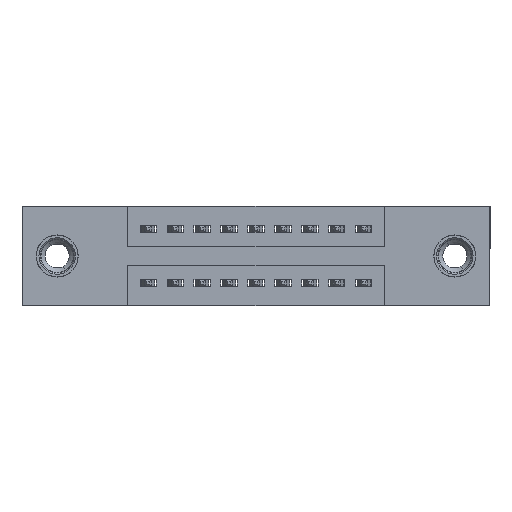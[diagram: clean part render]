
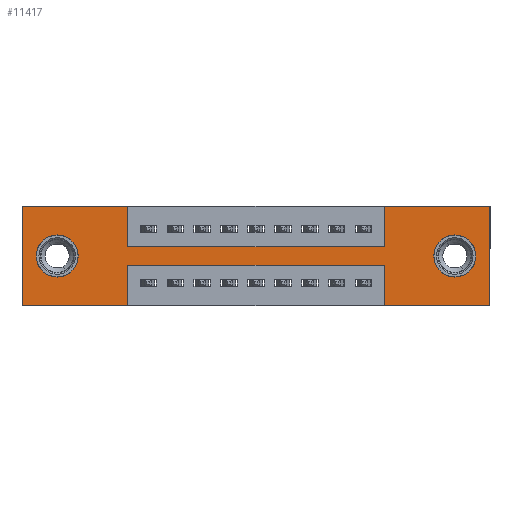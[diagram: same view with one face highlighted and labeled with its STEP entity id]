
A CAD part, front view. The second image highlights one B-rep face of the part: STEP entity #11417.
In plain terms, the highlighted planar face has unit normal (0, -1, 0).
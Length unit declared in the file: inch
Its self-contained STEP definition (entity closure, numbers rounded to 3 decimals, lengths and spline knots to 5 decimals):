
#374 = CARTESIAN_POINT ( 'NONE',  ( 0.13, 0., -0.263 ) ) ;
#575 = VERTEX_POINT ( 'NONE', #3489 ) ;
#651 = VERTEX_POINT ( 'NONE', #3044 ) ;
#823 = VERTEX_POINT ( 'NONE', #2618 ) ;
#985 = CARTESIAN_POINT ( 'NONE',  ( 1.3425, 0., 0. ) ) ;
#1018 = EDGE_CURVE ( 'NONE', #11412, #2988, #15150, .T. ) ;
#1039 = VERTEX_POINT ( 'NONE', #2217 ) ;
#1085 = EDGE_LOOP ( 'NONE', ( #7221, #8420 ) ) ;
#1152 = LINE ( 'NONE', #8568, #4815 ) ;
#1258 = CARTESIAN_POINT ( 'NONE',  ( 0., 0., -0.37 ) ) ;
#1342 = DIRECTION ( 'NONE',  ( 0., 0., 1. ) ) ;
#1344 = VERTEX_POINT ( 'NONE', #10447 ) ;
#1392 = DIRECTION ( 'NONE',  ( 0., 0., 1. ) ) ;
#1955 = VECTOR ( 'NONE', #10590, 39.37008 ) ;
#1995 = DIRECTION ( 'NONE',  ( 0., 1., 0. ) ) ;
#2217 = CARTESIAN_POINT ( 'NONE',  ( 0.3925, 0., -0.22 ) ) ;
#2341 = VERTEX_POINT ( 'NONE', #6808 ) ;
#2471 = FACE_BOUND ( 'NONE', #9876, .T. ) ;
#2543 = VERTEX_POINT ( 'NONE', #8246 ) ;
#2618 = CARTESIAN_POINT ( 'NONE',  ( 0., 0., 0. ) ) ;
#2703 = ORIENTED_EDGE ( 'NONE', *, *, #6531, .F. ) ;
#2709 = VERTEX_POINT ( 'NONE', #1258 ) ;
#2840 = LINE ( 'NONE', #4169, #12489 ) ;
#2851 = LINE ( 'NONE', #6890, #1955 ) ;
#2918 = VERTEX_POINT ( 'NONE', #7575 ) ;
#2976 = CARTESIAN_POINT ( 'NONE',  ( 0., 0., -0.37 ) ) ;
#2988 = VERTEX_POINT ( 'NONE', #10136 ) ;
#3044 = CARTESIAN_POINT ( 'NONE',  ( 1.735, 0., -0.37 ) ) ;
#3046 = VECTOR ( 'NONE', #15604, 39.37008 ) ;
#3374 = ORIENTED_EDGE ( 'NONE', *, *, #14021, .F. ) ;
#3489 = CARTESIAN_POINT ( 'NONE',  ( 1.605, 0., -0.107 ) ) ;
#3557 = ORIENTED_EDGE ( 'NONE', *, *, #7075, .T. ) ;
#3801 = CARTESIAN_POINT ( 'NONE',  ( 0.13, 0., -0.107 ) ) ;
#4063 = DIRECTION ( 'NONE',  ( 0., 0., -1. ) ) ;
#4169 = CARTESIAN_POINT ( 'NONE',  ( 0.3925, 0., -0.15 ) ) ;
#4176 = ORIENTED_EDGE ( 'NONE', *, *, #16287, .F. ) ;
#4330 = DIRECTION ( 'NONE',  ( 0., -1., 0. ) ) ;
#4395 = EDGE_CURVE ( 'NONE', #823, #2918, #2851, .T. ) ;
#4518 = VERTEX_POINT ( 'NONE', #374 ) ;
#4541 = VECTOR ( 'NONE', #7752, 39.37008 ) ;
#4552 = VECTOR ( 'NONE', #16025, 39.37008 ) ;
#4579 = EDGE_CURVE ( 'NONE', #2988, #1344, #10290, .T. ) ;
#4738 = EDGE_CURVE ( 'NONE', #2709, #823, #8368, .T. ) ;
#4815 = VECTOR ( 'NONE', #11016, 39.37008 ) ;
#4863 = EDGE_CURVE ( 'NONE', #2543, #11412, #2840, .T. ) ;
#5030 = CARTESIAN_POINT ( 'NONE',  ( 1.605, 0., -0.185 ) ) ;
#5120 = EDGE_CURVE ( 'NONE', #9756, #575, #8960, .T. ) ;
#5175 = DIRECTION ( 'NONE',  ( 0., 1., 0. ) ) ;
#5252 = CARTESIAN_POINT ( 'NONE',  ( 0., 0., -0.37 ) ) ;
#5296 = VERTEX_POINT ( 'NONE', #3801 ) ;
#5560 = VERTEX_POINT ( 'NONE', #9362 ) ;
#6025 = FACE_OUTER_BOUND ( 'NONE', #12438, .T. ) ;
#6253 = DIRECTION ( 'NONE',  ( 0., 0., -1. ) ) ;
#6317 = DIRECTION ( 'NONE',  ( 0., 0., -1. ) ) ;
#6364 = CARTESIAN_POINT ( 'NONE',  ( 1.3425, 0., -0.22 ) ) ;
#6531 = EDGE_CURVE ( 'NONE', #1344, #651, #11244, .T. ) ;
#6646 = ORIENTED_EDGE ( 'NONE', *, *, #1018, .F. ) ;
#6764 = CIRCLE ( 'NONE', #14622, 0.078 ) ;
#6808 = CARTESIAN_POINT ( 'NONE',  ( 1.3425, 0., -0.37 ) ) ;
#6890 = CARTESIAN_POINT ( 'NONE',  ( 0., 0., 0. ) ) ;
#7075 = EDGE_CURVE ( 'NONE', #4518, #5296, #6764, .T. ) ;
#7105 = CARTESIAN_POINT ( 'NONE',  ( 0.3925, 0., -0.37 ) ) ;
#7206 = DIRECTION ( 'NONE',  ( 1., 0., 0. ) ) ;
#7221 = ORIENTED_EDGE ( 'NONE', *, *, #12921, .T. ) ;
#7358 = EDGE_CURVE ( 'NONE', #10042, #1039, #15397, .T. ) ;
#7440 = ORIENTED_EDGE ( 'NONE', *, *, #4863, .F. ) ;
#7575 = CARTESIAN_POINT ( 'NONE',  ( 0.3925, 0., 0. ) ) ;
#7644 = ORIENTED_EDGE ( 'NONE', *, *, #4395, .F. ) ;
#7707 = LINE ( 'NONE', #9992, #15546 ) ;
#7752 = DIRECTION ( 'NONE',  ( 0., 0., 1. ) ) ;
#7918 = VECTOR ( 'NONE', #4063, 39.37008 ) ;
#7976 = LINE ( 'NONE', #13678, #10875 ) ;
#8048 = VECTOR ( 'NONE', #13817, 39.37008 ) ;
#8246 = CARTESIAN_POINT ( 'NONE',  ( 0.3925, 0., -0.15 ) ) ;
#8368 = LINE ( 'NONE', #13741, #4541 ) ;
#8420 = ORIENTED_EDGE ( 'NONE', *, *, #5120, .T. ) ;
#8480 = CARTESIAN_POINT ( 'NONE',  ( 0., 0., 0. ) ) ;
#8520 = EDGE_CURVE ( 'NONE', #1039, #5560, #11551, .T. ) ;
#8568 = CARTESIAN_POINT ( 'NONE',  ( 1.3425, 0., -0.37 ) ) ;
#8854 = AXIS2_PLACEMENT_3D ( 'NONE', #2976, #4330, #12988 ) ;
#8889 = ORIENTED_EDGE ( 'NONE', *, *, #12377, .F. ) ;
#8955 = CARTESIAN_POINT ( 'NONE',  ( 1.735, 0., 0. ) ) ;
#8960 = CIRCLE ( 'NONE', #15353, 0.078 ) ;
#9217 = DIRECTION ( 'NONE',  ( 0., 1., 0. ) ) ;
#9362 = CARTESIAN_POINT ( 'NONE',  ( 0.3925, 0., -0.37 ) ) ;
#9600 = ORIENTED_EDGE ( 'NONE', *, *, #4579, .F. ) ;
#9633 = CARTESIAN_POINT ( 'NONE',  ( 1.605, 0., -0.263 ) ) ;
#9756 = VERTEX_POINT ( 'NONE', #9633 ) ;
#9800 = CARTESIAN_POINT ( 'NONE',  ( 1.605, 0., -0.185 ) ) ;
#9876 = EDGE_LOOP ( 'NONE', ( #15468, #3557 ) ) ;
#9992 = CARTESIAN_POINT ( 'NONE',  ( 0.3925, 0., 0. ) ) ;
#10042 = VERTEX_POINT ( 'NONE', #6364 ) ;
#10136 = CARTESIAN_POINT ( 'NONE',  ( 1.3425, 0., 0. ) ) ;
#10290 = LINE ( 'NONE', #8480, #13044 ) ;
#10393 = EDGE_CURVE ( 'NONE', #2341, #10042, #1152, .T. ) ;
#10447 = CARTESIAN_POINT ( 'NONE',  ( 1.735, 0., 0. ) ) ;
#10590 = DIRECTION ( 'NONE',  ( 1., 0., 0. ) ) ;
#10650 = PLANE ( 'NONE',  #8854 ) ;
#10735 = ORIENTED_EDGE ( 'NONE', *, *, #8520, .F. ) ;
#10875 = VECTOR ( 'NONE', #12507, 39.37008 ) ;
#11016 = DIRECTION ( 'NONE',  ( 0., 0., 1. ) ) ;
#11050 = DIRECTION ( 'NONE',  ( 0., 0., -1. ) ) ;
#11117 = ORIENTED_EDGE ( 'NONE', *, *, #7358, .F. ) ;
#11244 = LINE ( 'NONE', #8955, #4552 ) ;
#11412 = VERTEX_POINT ( 'NONE', #14148 ) ;
#11417 = ADVANCED_FACE ( 'NONE', ( #15648, #2471, #6025 ), #10650, .T. ) ;
#11551 = LINE ( 'NONE', #7105, #7918 ) ;
#11675 = LINE ( 'NONE', #5252, #8048 ) ;
#11721 = DIRECTION ( 'NONE',  ( 1., 0., 0. ) ) ;
#12072 = VECTOR ( 'NONE', #1392, 39.37008 ) ;
#12377 = EDGE_CURVE ( 'NONE', #5560, #2709, #7976, .T. ) ;
#12411 = AXIS2_PLACEMENT_3D ( 'NONE', #12581, #5175, #13754 ) ;
#12438 = EDGE_LOOP ( 'NONE', ( #10735, #11117, #14933, #4176, #2703, #9600, #6646, #7440, #3374, #7644, #15535, #8889 ) ) ;
#12489 = VECTOR ( 'NONE', #11721, 39.37008 ) ;
#12507 = DIRECTION ( 'NONE',  ( -1., 0., 0. ) ) ;
#12581 = CARTESIAN_POINT ( 'NONE',  ( 0.13, 0., -0.185 ) ) ;
#12921 = EDGE_CURVE ( 'NONE', #575, #9756, #16295, .T. ) ;
#12988 = DIRECTION ( 'NONE',  ( 0., 0., -1. ) ) ;
#13044 = VECTOR ( 'NONE', #7206, 39.37008 ) ;
#13416 = EDGE_CURVE ( 'NONE', #5296, #4518, #15200, .T. ) ;
#13604 = DIRECTION ( 'NONE',  ( 0., 1., 0. ) ) ;
#13678 = CARTESIAN_POINT ( 'NONE',  ( 0., 0., -0.37 ) ) ;
#13741 = CARTESIAN_POINT ( 'NONE',  ( 0., 0., 0. ) ) ;
#13754 = DIRECTION ( 'NONE',  ( 0., 0., 1. ) ) ;
#13817 = DIRECTION ( 'NONE',  ( -1., 0., 0. ) ) ;
#14021 = EDGE_CURVE ( 'NONE', #2918, #2543, #7707, .T. ) ;
#14148 = CARTESIAN_POINT ( 'NONE',  ( 1.3425, 0., -0.15 ) ) ;
#14574 = AXIS2_PLACEMENT_3D ( 'NONE', #5030, #13604, #6317 ) ;
#14619 = CARTESIAN_POINT ( 'NONE',  ( 0.3925, 0., -0.22 ) ) ;
#14622 = AXIS2_PLACEMENT_3D ( 'NONE', #16269, #9217, #1342 ) ;
#14933 = ORIENTED_EDGE ( 'NONE', *, *, #10393, .F. ) ;
#15150 = LINE ( 'NONE', #985, #12072 ) ;
#15200 = CIRCLE ( 'NONE', #12411, 0.078 ) ;
#15353 = AXIS2_PLACEMENT_3D ( 'NONE', #9800, #1995, #11050 ) ;
#15397 = LINE ( 'NONE', #14619, #3046 ) ;
#15468 = ORIENTED_EDGE ( 'NONE', *, *, #13416, .T. ) ;
#15535 = ORIENTED_EDGE ( 'NONE', *, *, #4738, .F. ) ;
#15546 = VECTOR ( 'NONE', #6253, 39.37008 ) ;
#15604 = DIRECTION ( 'NONE',  ( -1., 0., 0. ) ) ;
#15648 = FACE_BOUND ( 'NONE', #1085, .T. ) ;
#16025 = DIRECTION ( 'NONE',  ( 0., 0., -1. ) ) ;
#16269 = CARTESIAN_POINT ( 'NONE',  ( 0.13, 0., -0.185 ) ) ;
#16287 = EDGE_CURVE ( 'NONE', #651, #2341, #11675, .T. ) ;
#16295 = CIRCLE ( 'NONE', #14574, 0.078 ) ;
